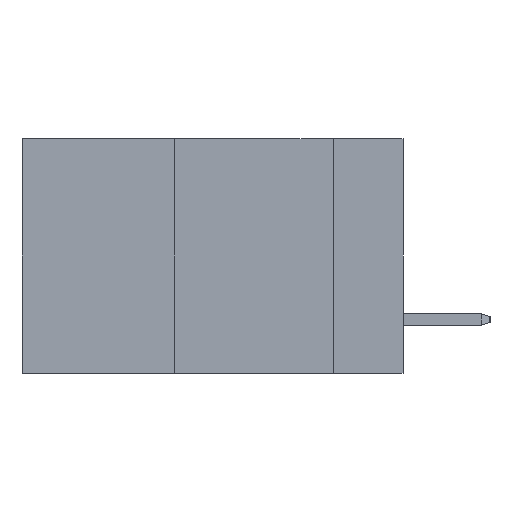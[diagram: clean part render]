
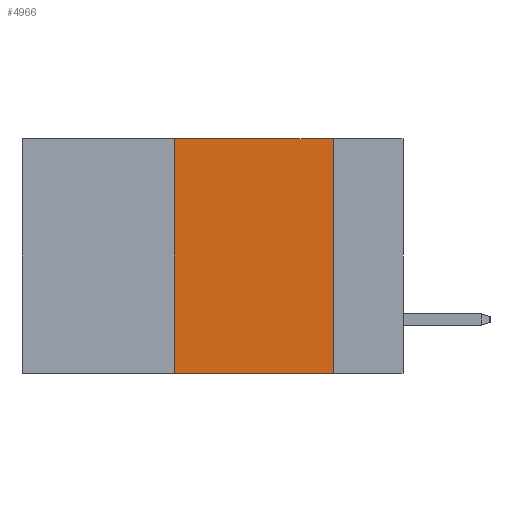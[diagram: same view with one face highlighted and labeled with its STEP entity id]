
A CAD part, left-side view. The second image highlights one B-rep face of the part: STEP entity #4966.
In plain terms, the highlighted planar face has unit normal (-1, 0, 0).
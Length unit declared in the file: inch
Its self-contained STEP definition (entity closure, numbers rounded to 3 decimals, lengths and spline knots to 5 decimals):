
#878 = ORIENTED_EDGE ( 'NONE', *, *, #7853, .F. ) ;
#1860 = VERTEX_POINT ( 'NONE', #11148 ) ;
#1905 = CARTESIAN_POINT ( 'NONE',  ( 0., 0.36, 0. ) ) ;
#1961 = CARTESIAN_POINT ( 'NONE',  ( 0., 0.11, -0.37 ) ) ;
#2109 = VERTEX_POINT ( 'NONE', #3010 ) ;
#2619 = EDGE_CURVE ( 'NONE', #1860, #4271, #4788, .T. ) ;
#3010 = CARTESIAN_POINT ( 'NONE',  ( 0., 0.36, 0. ) ) ;
#4037 = FACE_OUTER_BOUND ( 'NONE', #5884, .T. ) ;
#4117 = EDGE_CURVE ( 'NONE', #12158, #4271, #8680, .T. ) ;
#4221 = DIRECTION ( 'NONE',  ( 0., 0., 1. ) ) ;
#4271 = VERTEX_POINT ( 'NONE', #1961 ) ;
#4472 = EDGE_CURVE ( 'NONE', #1860, #2109, #9569, .T. ) ;
#4788 = LINE ( 'NONE', #9334, #13471 ) ;
#4966 = ADVANCED_FACE ( 'NONE', ( #4037 ), #9977, .F. ) ;
#5074 = VECTOR ( 'NONE', #4221, 39.37008 ) ;
#5884 = EDGE_LOOP ( 'NONE', ( #14100, #878, #6598, #8582 ) ) ;
#5971 = DIRECTION ( 'NONE',  ( 0., -1., 0. ) ) ;
#6492 = CARTESIAN_POINT ( 'NONE',  ( 0., 0.11, 0. ) ) ;
#6598 = ORIENTED_EDGE ( 'NONE', *, *, #4472, .F. ) ;
#7223 = LINE ( 'NONE', #11688, #8211 ) ;
#7541 = CARTESIAN_POINT ( 'NONE',  ( 0., 0.6, 0. ) ) ;
#7853 = EDGE_CURVE ( 'NONE', #2109, #12158, #7223, .T. ) ;
#8211 = VECTOR ( 'NONE', #9526, 39.37008 ) ;
#8582 = ORIENTED_EDGE ( 'NONE', *, *, #2619, .T. ) ;
#8603 = DIRECTION ( 'NONE',  ( 0., 0., -1. ) ) ;
#8680 = LINE ( 'NONE', #14128, #11639 ) ;
#9334 = CARTESIAN_POINT ( 'NONE',  ( 0., 0.6, -0.37 ) ) ;
#9526 = DIRECTION ( 'NONE',  ( 0., -1., 0. ) ) ;
#9569 = LINE ( 'NONE', #1905, #5074 ) ;
#9977 = PLANE ( 'NONE',  #13239 ) ;
#11148 = CARTESIAN_POINT ( 'NONE',  ( 0., 0.36, -0.37 ) ) ;
#11639 = VECTOR ( 'NONE', #8603, 39.37008 ) ;
#11688 = CARTESIAN_POINT ( 'NONE',  ( 0., 0.6, 0. ) ) ;
#12002 = DIRECTION ( 'NONE',  ( 0., 0., -1. ) ) ;
#12158 = VERTEX_POINT ( 'NONE', #6492 ) ;
#13239 = AXIS2_PLACEMENT_3D ( 'NONE', #7541, #14333, #12002 ) ;
#13471 = VECTOR ( 'NONE', #5971, 39.37008 ) ;
#14100 = ORIENTED_EDGE ( 'NONE', *, *, #4117, .F. ) ;
#14128 = CARTESIAN_POINT ( 'NONE',  ( 0., 0.11, 0. ) ) ;
#14333 = DIRECTION ( 'NONE',  ( 1., 0., 0. ) ) ;
